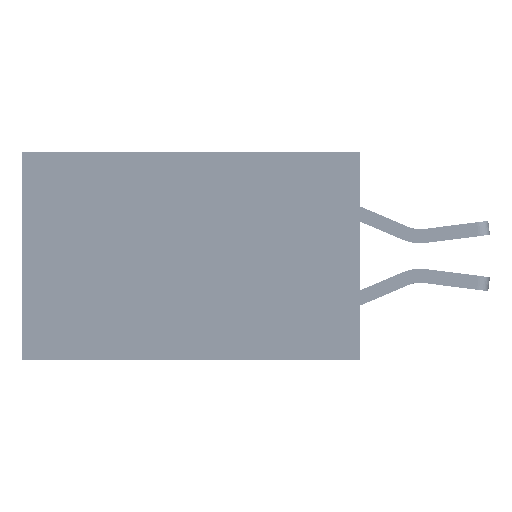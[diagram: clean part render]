
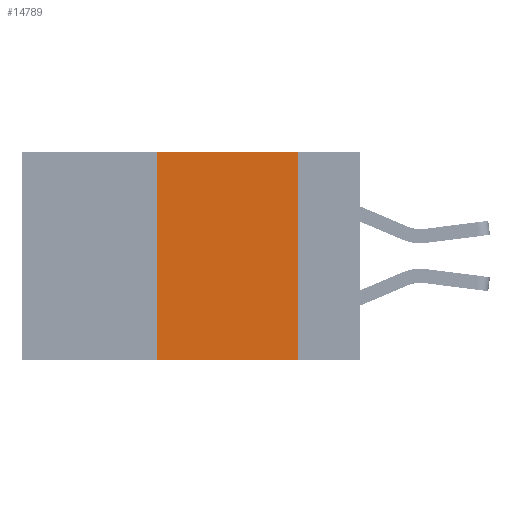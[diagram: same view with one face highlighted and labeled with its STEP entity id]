
A CAD part, left-side view. The second image highlights one B-rep face of the part: STEP entity #14789.
In plain terms, the highlighted planar face has unit normal (-1, 0, 0).
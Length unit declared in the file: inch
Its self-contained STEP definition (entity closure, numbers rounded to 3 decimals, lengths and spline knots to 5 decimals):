
#863 = VECTOR ( 'NONE', #17164, 39.37008 ) ;
#2874 = CARTESIAN_POINT ( 'NONE',  ( 0., 0.36, 0. ) ) ;
#3105 = AXIS2_PLACEMENT_3D ( 'NONE', #30901, #16422, #36801 ) ;
#3507 = EDGE_CURVE ( 'NONE', #17606, #32320, #35074, .T. ) ;
#4558 = ORIENTED_EDGE ( 'NONE', *, *, #8612, .T. ) ;
#7997 = FACE_OUTER_BOUND ( 'NONE', #18179, .T. ) ;
#8612 = EDGE_CURVE ( 'NONE', #17606, #14436, #16376, .T. ) ;
#8757 = DIRECTION ( 'NONE',  ( 0., 0., -1. ) ) ;
#9375 = ORIENTED_EDGE ( 'NONE', *, *, #13362, .F. ) ;
#10598 = LINE ( 'NONE', #31971, #12410 ) ;
#12410 = VECTOR ( 'NONE', #8757, 39.37008 ) ;
#12669 = DIRECTION ( 'NONE',  ( 0., 0., 1. ) ) ;
#13362 = EDGE_CURVE ( 'NONE', #34939, #14436, #10598, .T. ) ;
#14436 = VERTEX_POINT ( 'NONE', #14625 ) ;
#14625 = CARTESIAN_POINT ( 'NONE',  ( 0., 0.11, -0.37 ) ) ;
#14789 = ADVANCED_FACE ( 'NONE', ( #7997 ), #16548, .F. ) ;
#15510 = ORIENTED_EDGE ( 'NONE', *, *, #3507, .F. ) ;
#16376 = LINE ( 'NONE', #31427, #32568 ) ;
#16422 = DIRECTION ( 'NONE',  ( 1., 0., 0. ) ) ;
#16548 = PLANE ( 'NONE',  #3105 ) ;
#17164 = DIRECTION ( 'NONE',  ( 0., -1., 0. ) ) ;
#17606 = VERTEX_POINT ( 'NONE', #18835 ) ;
#18179 = EDGE_LOOP ( 'NONE', ( #9375, #23891, #15510, #4558 ) ) ;
#18835 = CARTESIAN_POINT ( 'NONE',  ( 0., 0.36, -0.37 ) ) ;
#18834 = LINE ( 'NONE', #21791, #863 ) ;
#20000 = CARTESIAN_POINT ( 'NONE',  ( 0., 0.11, 0. ) ) ;
#21791 = CARTESIAN_POINT ( 'NONE',  ( 0., 0.6, 0. ) ) ;
#23864 = EDGE_CURVE ( 'NONE', #32320, #34939, #18834, .T. ) ;
#23891 = ORIENTED_EDGE ( 'NONE', *, *, #23864, .F. ) ;
#25047 = VECTOR ( 'NONE', #12669, 39.37008 ) ;
#30061 = CARTESIAN_POINT ( 'NONE',  ( 0., 0.36, 0. ) ) ;
#30901 = CARTESIAN_POINT ( 'NONE',  ( 0., 0.6, 0. ) ) ;
#31171 = DIRECTION ( 'NONE',  ( 0., -1., 0. ) ) ;
#31427 = CARTESIAN_POINT ( 'NONE',  ( 0., 0.6, -0.37 ) ) ;
#31971 = CARTESIAN_POINT ( 'NONE',  ( 0., 0.11, 0. ) ) ;
#32320 = VERTEX_POINT ( 'NONE', #2874 ) ;
#32568 = VECTOR ( 'NONE', #31171, 39.37008 ) ;
#34939 = VERTEX_POINT ( 'NONE', #20000 ) ;
#35074 = LINE ( 'NONE', #30061, #25047 ) ;
#36801 = DIRECTION ( 'NONE',  ( 0., 0., -1. ) ) ;
